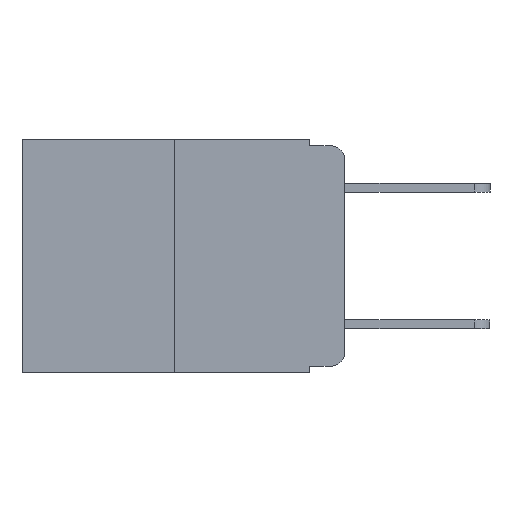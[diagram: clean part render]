
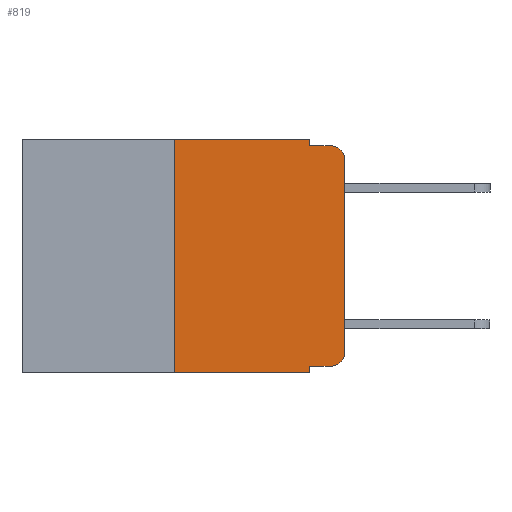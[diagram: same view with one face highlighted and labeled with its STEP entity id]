
A CAD part, left-side view. The second image highlights one B-rep face of the part: STEP entity #819.
In plain terms, the highlighted planar face has unit normal (-1, 0, 0).
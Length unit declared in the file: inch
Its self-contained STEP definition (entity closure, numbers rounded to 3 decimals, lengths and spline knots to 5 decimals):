
#120 = VERTEX_POINT ( 'NONE', #1834 ) ;
#498 = DIRECTION ( 'NONE',  ( 0., 0., 1. ) ) ;
#505 = VERTEX_POINT ( 'NONE', #4144 ) ;
#819 = ADVANCED_FACE ( 'NONE', ( #11360 ), #7792, .F. ) ;
#1158 = AXIS2_PLACEMENT_3D ( 'NONE', #12773, #10746, #2339 ) ;
#1414 = CARTESIAN_POINT ( 'NONE',  ( 0., 0.051, 0. ) ) ;
#1486 = ORIENTED_EDGE ( 'NONE', *, *, #1609, .F. ) ;
#1607 = CARTESIAN_POINT ( 'NONE',  ( 0., 0.051, -0.343 ) ) ;
#1609 = EDGE_CURVE ( 'NONE', #120, #10466, #8736, .T. ) ;
#1632 = LINE ( 'NONE', #8650, #9721 ) ;
#1834 = CARTESIAN_POINT ( 'NONE',  ( 0., 0.25, 0. ) ) ;
#1869 = LINE ( 'NONE', #5067, #7609 ) ;
#2080 = EDGE_CURVE ( 'NONE', #7907, #8365, #1869, .T. ) ;
#2180 = ORIENTED_EDGE ( 'NONE', *, *, #2823, .F. ) ;
#2204 = ORIENTED_EDGE ( 'NONE', *, *, #2868, .T. ) ;
#2339 = DIRECTION ( 'NONE',  ( 0., 0., -1. ) ) ;
#2758 = EDGE_CURVE ( 'NONE', #10602, #4095, #1632, .T. ) ;
#2797 = EDGE_CURVE ( 'NONE', #4095, #10814, #9127, .T. ) ;
#2820 = EDGE_CURVE ( 'NONE', #8185, #10814, #12712, .T. ) ;
#2823 = EDGE_CURVE ( 'NONE', #10466, #8185, #8530, .T. ) ;
#2838 = DIRECTION ( 'NONE',  ( -1., 0., 0. ) ) ;
#2844 = EDGE_CURVE ( 'NONE', #7907, #120, #12406, .T. ) ;
#2847 = EDGE_CURVE ( 'NONE', #505, #8365, #5207, .T. ) ;
#2865 = EDGE_CURVE ( 'NONE', #505, #7677, #4579, .T. ) ;
#2868 = EDGE_CURVE ( 'NONE', #7677, #10602, #11910, .T. ) ;
#3679 = CARTESIAN_POINT ( 'NONE',  ( 0., 0.473, 0. ) ) ;
#3950 = CARTESIAN_POINT ( 'NONE',  ( 0., 0., -0.313 ) ) ;
#4013 = DIRECTION ( 'NONE',  ( 0., 0., -1. ) ) ;
#4095 = VERTEX_POINT ( 'NONE', #6791 ) ;
#4144 = CARTESIAN_POINT ( 'NONE',  ( 0., 0.051, -0.333 ) ) ;
#4579 = LINE ( 'NONE', #5259, #9873 ) ;
#4908 = VECTOR ( 'NONE', #498, 39.37008 ) ;
#5067 = CARTESIAN_POINT ( 'NONE',  ( 0., 0.473, -0.343 ) ) ;
#5207 = LINE ( 'NONE', #11837, #12161 ) ;
#5259 = CARTESIAN_POINT ( 'NONE',  ( 0., 0.051, -0.333 ) ) ;
#5266 = ORIENTED_EDGE ( 'NONE', *, *, #2820, .F. ) ;
#5349 = DIRECTION ( 'NONE',  ( -1., 0., 0. ) ) ;
#5621 = AXIS2_PLACEMENT_3D ( 'NONE', #9075, #2838, #4013 ) ;
#5827 = VECTOR ( 'NONE', #8908, 39.37008 ) ;
#6215 = DIRECTION ( 'NONE',  ( 0., 0., -1. ) ) ;
#6399 = CARTESIAN_POINT ( 'NONE',  ( 0., 0.02, -0.03 ) ) ;
#6509 = VECTOR ( 'NONE', #9508, 39.37008 ) ;
#6791 = CARTESIAN_POINT ( 'NONE',  ( 0., 0., -0.03 ) ) ;
#6821 = CARTESIAN_POINT ( 'NONE',  ( 0., 0.051, -0.01 ) ) ;
#7150 = EDGE_LOOP ( 'NONE', ( #11531, #11165, #5266, #2180, #1486, #7711, #11098, #12760, #7411, #2204 ) ) ;
#7411 = ORIENTED_EDGE ( 'NONE', *, *, #2865, .T. ) ;
#7609 = VECTOR ( 'NONE', #11193, 39.37008 ) ;
#7677 = VERTEX_POINT ( 'NONE', #9240 ) ;
#7711 = ORIENTED_EDGE ( 'NONE', *, *, #2844, .F. ) ;
#7792 = PLANE ( 'NONE',  #1158 ) ;
#7907 = VERTEX_POINT ( 'NONE', #12087 ) ;
#8185 = VERTEX_POINT ( 'NONE', #11496 ) ;
#8365 = VERTEX_POINT ( 'NONE', #1607 ) ;
#8530 = LINE ( 'NONE', #1414, #5827 ) ;
#8650 = CARTESIAN_POINT ( 'NONE',  ( 0., 0., 0. ) ) ;
#8736 = LINE ( 'NONE', #3679, #10607 ) ;
#8908 = DIRECTION ( 'NONE',  ( 0., 0., -1. ) ) ;
#8960 = DIRECTION ( 'NONE',  ( 0., -1., 0. ) ) ;
#9075 = CARTESIAN_POINT ( 'NONE',  ( 0., 0.02, -0.313 ) ) ;
#9127 = CIRCLE ( 'NONE', #12701, 0.02 ) ;
#9240 = CARTESIAN_POINT ( 'NONE',  ( 0., 0.02, -0.333 ) ) ;
#9508 = DIRECTION ( 'NONE',  ( 0., -1., 0. ) ) ;
#9721 = VECTOR ( 'NONE', #12116, 39.37008 ) ;
#9873 = VECTOR ( 'NONE', #8960, 39.37008 ) ;
#10135 = CARTESIAN_POINT ( 'NONE',  ( 0., 0.25, 0. ) ) ;
#10466 = VERTEX_POINT ( 'NONE', #12423 ) ;
#10602 = VERTEX_POINT ( 'NONE', #3950 ) ;
#10607 = VECTOR ( 'NONE', #12072, 39.37008 ) ;
#10746 = DIRECTION ( 'NONE',  ( 1., 0., 0. ) ) ;
#10814 = VERTEX_POINT ( 'NONE', #12686 ) ;
#11098 = ORIENTED_EDGE ( 'NONE', *, *, #2080, .T. ) ;
#11165 = ORIENTED_EDGE ( 'NONE', *, *, #2797, .T. ) ;
#11193 = DIRECTION ( 'NONE',  ( 0., -1., 0. ) ) ;
#11325 = DIRECTION ( 'NONE',  ( 0., 0., -1. ) ) ;
#11360 = FACE_OUTER_BOUND ( 'NONE', #7150, .T. ) ;
#11496 = CARTESIAN_POINT ( 'NONE',  ( 0., 0.051, -0.01 ) ) ;
#11531 = ORIENTED_EDGE ( 'NONE', *, *, #2758, .T. ) ;
#11837 = CARTESIAN_POINT ( 'NONE',  ( 0., 0.051, 0. ) ) ;
#11910 = CIRCLE ( 'NONE', #5621, 0.02 ) ;
#12072 = DIRECTION ( 'NONE',  ( 0., -1., 0. ) ) ;
#12087 = CARTESIAN_POINT ( 'NONE',  ( 0., 0.25, -0.343 ) ) ;
#12116 = DIRECTION ( 'NONE',  ( 0., 0., 1. ) ) ;
#12161 = VECTOR ( 'NONE', #11325, 39.37008 ) ;
#12406 = LINE ( 'NONE', #10135, #4908 ) ;
#12423 = CARTESIAN_POINT ( 'NONE',  ( 0., 0.051, 0. ) ) ;
#12686 = CARTESIAN_POINT ( 'NONE',  ( 0., 0.02, -0.01 ) ) ;
#12701 = AXIS2_PLACEMENT_3D ( 'NONE', #6399, #5349, #6215 ) ;
#12712 = LINE ( 'NONE', #6821, #6509 ) ;
#12760 = ORIENTED_EDGE ( 'NONE', *, *, #2847, .F. ) ;
#12773 = CARTESIAN_POINT ( 'NONE',  ( 0., 0.473, 0. ) ) ;
